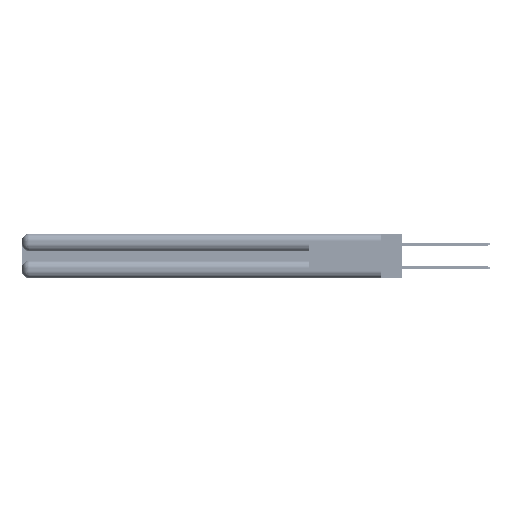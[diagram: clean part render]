
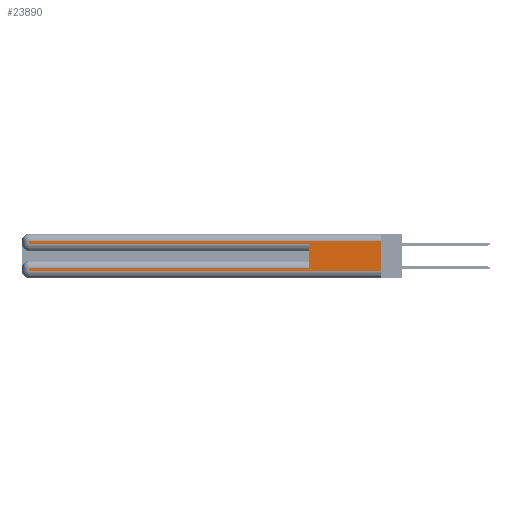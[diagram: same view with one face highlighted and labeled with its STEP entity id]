
A CAD part, left-side view. The second image highlights one B-rep face of the part: STEP entity #23890.
In plain terms, the highlighted planar face has unit normal (-1, 0, 0).
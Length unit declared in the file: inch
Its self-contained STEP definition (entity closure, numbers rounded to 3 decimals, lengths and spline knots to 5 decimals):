
#1609 = VERTEX_POINT ( 'NONE', #5330 ) ;
#1861 = EDGE_CURVE ( 'NONE', #46161, #6910, #31971, .T. ) ;
#2252 = CARTESIAN_POINT ( 'NONE',  ( 0., 2.94, 0.085 ) ) ;
#3467 = DIRECTION ( 'NONE',  ( 0., 1., 0. ) ) ;
#3617 = CARTESIAN_POINT ( 'NONE',  ( 0., 0.6, 0.145 ) ) ;
#3809 = CARTESIAN_POINT ( 'NONE',  ( 0., 0., 0.06 ) ) ;
#4590 = CARTESIAN_POINT ( 'NONE',  ( 0., 2.94, 0.06 ) ) ;
#4685 = VECTOR ( 'NONE', #3467, 39.37008 ) ;
#4709 = VECTOR ( 'NONE', #32212, 39.37008 ) ;
#5330 = CARTESIAN_POINT ( 'NONE',  ( 0., 0.6, 0.285 ) ) ;
#6366 = CARTESIAN_POINT ( 'NONE',  ( 0., 0., 0.31 ) ) ;
#6910 = VERTEX_POINT ( 'NONE', #2252 ) ;
#8655 = DIRECTION ( 'NONE',  ( 0., 0., -1. ) ) ;
#10336 = VERTEX_POINT ( 'NONE', #55390 ) ;
#10431 = ORIENTED_EDGE ( 'NONE', *, *, #1861, .T. ) ;
#11236 = LINE ( 'NONE', #52958, #30317 ) ;
#11578 = DIRECTION ( 'NONE',  ( 0., -1., 0. ) ) ;
#12061 = VERTEX_POINT ( 'NONE', #45534 ) ;
#12122 = VERTEX_POINT ( 'NONE', #6366 ) ;
#16945 = LINE ( 'NONE', #3617, #46373 ) ;
#18967 = DIRECTION ( 'NONE',  ( 0., 0., -1. ) ) ;
#20149 = CARTESIAN_POINT ( 'NONE',  ( 0., 0., 0.285 ) ) ;
#20848 = AXIS2_PLACEMENT_3D ( 'NONE', #43811, #48227, #52590 ) ;
#21801 = EDGE_CURVE ( 'NONE', #46161, #1609, #16945, .T. ) ;
#23890 = ADVANCED_FACE ( 'NONE', ( #52891 ), #39554, .F. ) ;
#24044 = ORIENTED_EDGE ( 'NONE', *, *, #30768, .F. ) ;
#24658 = VERTEX_POINT ( 'NONE', #4590 ) ;
#24678 = EDGE_CURVE ( 'NONE', #12061, #45602, #31316, .T. ) ;
#25270 = LINE ( 'NONE', #3809, #48539 ) ;
#26706 = ORIENTED_EDGE ( 'NONE', *, *, #33101, .T. ) ;
#26784 = EDGE_CURVE ( 'NONE', #6910, #24658, #11236, .T. ) ;
#29033 = VECTOR ( 'NONE', #18967, 39.37008 ) ;
#29156 = DIRECTION ( 'NONE',  ( 0., 1., 0. ) ) ;
#30317 = VECTOR ( 'NONE', #8655, 39.37008 ) ;
#30768 = EDGE_CURVE ( 'NONE', #12122, #10336, #53697, .T. ) ;
#31316 = LINE ( 'NONE', #40448, #4709 ) ;
#31971 = LINE ( 'NONE', #33531, #49797 ) ;
#32212 = DIRECTION ( 'NONE',  ( 0., 0., -1. ) ) ;
#33101 = EDGE_CURVE ( 'NONE', #24658, #10336, #25270, .T. ) ;
#33531 = CARTESIAN_POINT ( 'NONE',  ( 0., 0., 0.085 ) ) ;
#35382 = LINE ( 'NONE', #55766, #4685 ) ;
#37600 = EDGE_CURVE ( 'NONE', #45602, #1609, #40249, .T. ) ;
#37838 = ORIENTED_EDGE ( 'NONE', *, *, #26784, .T. ) ;
#38626 = ORIENTED_EDGE ( 'NONE', *, *, #37600, .T. ) ;
#38701 = DIRECTION ( 'NONE',  ( 0., -1., 0. ) ) ;
#39554 = PLANE ( 'NONE',  #20848 ) ;
#39649 = EDGE_LOOP ( 'NONE', ( #24044, #55733, #44861, #38626, #42834, #10431, #37838, #26706 ) ) ;
#40249 = LINE ( 'NONE', #20149, #51139 ) ;
#40448 = CARTESIAN_POINT ( 'NONE',  ( 0., 2.94, 0.37 ) ) ;
#42834 = ORIENTED_EDGE ( 'NONE', *, *, #21801, .F. ) ;
#43811 = CARTESIAN_POINT ( 'NONE',  ( 0., 0., 0.37 ) ) ;
#44861 = ORIENTED_EDGE ( 'NONE', *, *, #24678, .T. ) ;
#45534 = CARTESIAN_POINT ( 'NONE',  ( 0., 2.94, 0.31 ) ) ;
#45602 = VERTEX_POINT ( 'NONE', #51917 ) ;
#46161 = VERTEX_POINT ( 'NONE', #51297 ) ;
#46373 = VECTOR ( 'NONE', #51548, 39.37008 ) ;
#48227 = DIRECTION ( 'NONE',  ( 1., 0., 0. ) ) ;
#48539 = VECTOR ( 'NONE', #38701, 39.37008 ) ;
#49797 = VECTOR ( 'NONE', #29156, 39.37008 ) ;
#49903 = EDGE_CURVE ( 'NONE', #12122, #12061, #35382, .T. ) ;
#50127 = CARTESIAN_POINT ( 'NONE',  ( 0., 0., 0.37 ) ) ;
#51139 = VECTOR ( 'NONE', #11578, 39.37008 ) ;
#51297 = CARTESIAN_POINT ( 'NONE',  ( 0., 0.6, 0.085 ) ) ;
#51548 = DIRECTION ( 'NONE',  ( 0., 0., 1. ) ) ;
#51917 = CARTESIAN_POINT ( 'NONE',  ( 0., 2.94, 0.285 ) ) ;
#52590 = DIRECTION ( 'NONE',  ( 0., 0., -1. ) ) ;
#52891 = FACE_OUTER_BOUND ( 'NONE', #39649, .T. ) ;
#52958 = CARTESIAN_POINT ( 'NONE',  ( 0., 2.94, 0.37 ) ) ;
#53697 = LINE ( 'NONE', #50127, #29033 ) ;
#55390 = CARTESIAN_POINT ( 'NONE',  ( 0., 0., 0.06 ) ) ;
#55733 = ORIENTED_EDGE ( 'NONE', *, *, #49903, .T. ) ;
#55766 = CARTESIAN_POINT ( 'NONE',  ( 0., 0., 0.31 ) ) ;
